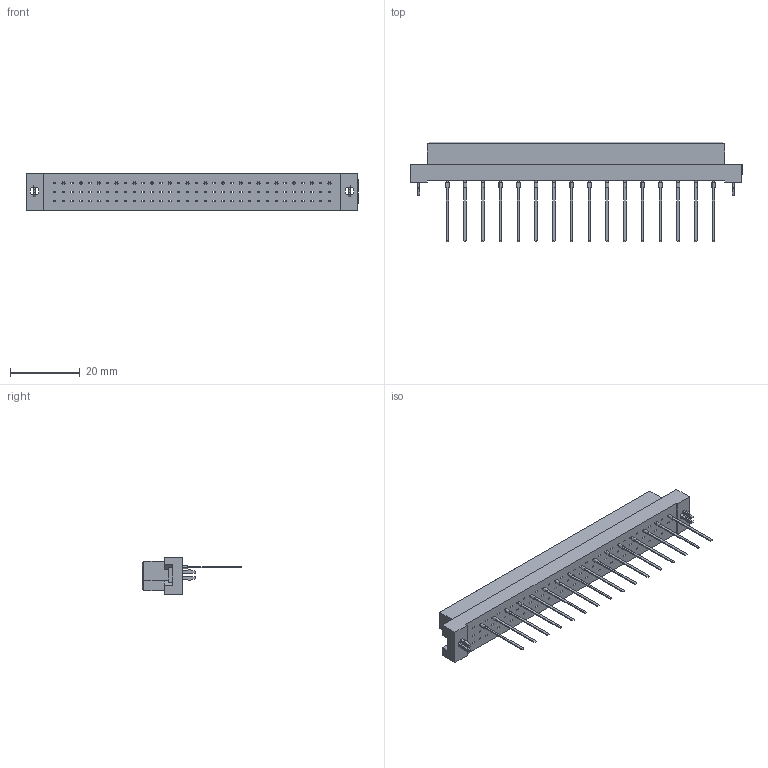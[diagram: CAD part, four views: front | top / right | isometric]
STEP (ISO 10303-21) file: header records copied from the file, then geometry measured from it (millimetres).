
FILE_DESCRIPTION (( 'STEP AP203' ), '1' );
FILE_NAME ('496-116-381-123.STEP', '2019-11-12T12:57:47', ( '' ), ( '' ), 'SwSTEP 2.0', 'SolidWorks 2020', '' );
FILE_SCHEMA (( 'CONFIG_CONTROL_DESIGN' ));
Length unit declared in the file: millimetre
Products named in the file (4): 496 Part_96; 496 Bore-lock; 496-116-381-123; 496-290_81
Assembly tree (19 placements, depth 2):
  496-116-381-123
    496 Part_96
    496-290_81  x16
    496 Bore-lock  x2
Bounding box: 95 x 28.6 x 10.6 mm (x, y, z)
Volume: 106.9 mm3
Topology: 18 solids, 22 shells, 1614 faces, 3886 edges, 2440 vertices
Faces by surface type: plane 1576, cylinder 38
Entity records: 39130 total; most frequent: CARTESIAN_POINT 6664, ORIENTED_EDGE 6540, DIRECTION 5978, EDGE_CURVE 3270, VECTOR 3254, LINE 3254, VERTEX_POINT 2048, EDGE_LOOP 1620
